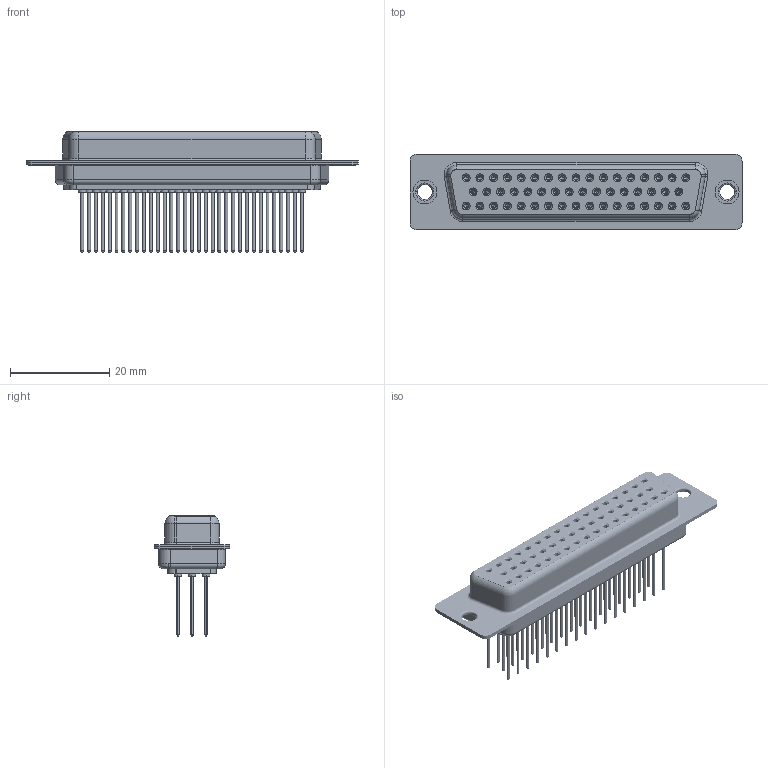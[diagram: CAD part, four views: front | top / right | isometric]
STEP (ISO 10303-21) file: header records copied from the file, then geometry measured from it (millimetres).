
FILE_DESCRIPTION (( 'STEP AP203' ), '1' );
FILE_NAME ('628-M50-623-WT1.STEP', '2020-07-17T10:45:24', ( '' ), ( '' ), 'SwSTEP 2.0', 'SolidWorks 2020', '' );
FILE_SCHEMA (( 'CONFIG_CONTROL_DESIGN' ));
Length unit declared in the file: millimetre
Products named in the file (8): 628M Shell Front_50 Contacts; 628M Thru Hole Rivet; 628M Contact Row 1_23; 628M Contact Row 2_23; 628-M50-623-WT1; 628M Contact Row 3_23; 628M Shell Rear_50 Contacts; 628M Housing_50 Contacts
Assembly tree (55 placements, depth 2):
  628-M50-623-WT1
    628M Housing_50 Contacts
    628M Shell Front_50 Contacts
    628M Shell Rear_50 Contacts
    628M Contact Row 1_23  x17
    628M Contact Row 2_23  x16
    628M Contact Row 3_23  x17
    628M Thru Hole Rivet  x2
Bounding box: 67 x 15.3 x 24.27 mm (x, y, z)
Volume: 6638.2 mm3; surface area: 15521.4 mm2
Topology: 55 solids, 55 shells, 3003 faces, 6903 edges, 4221 vertices
Faces by surface type: cylinder 1071, plane 817, torus 765, cone 350
Entity records: 31140 total; most frequent: DIRECTION 5679, CARTESIAN_POINT 4998, ORIENTED_EDGE 4502, AXIS2_PLACEMENT_3D 2430, EDGE_CURVE 2251, VERTEX_POINT 1424, CIRCLE 1363, EDGE_LOOP 1291
